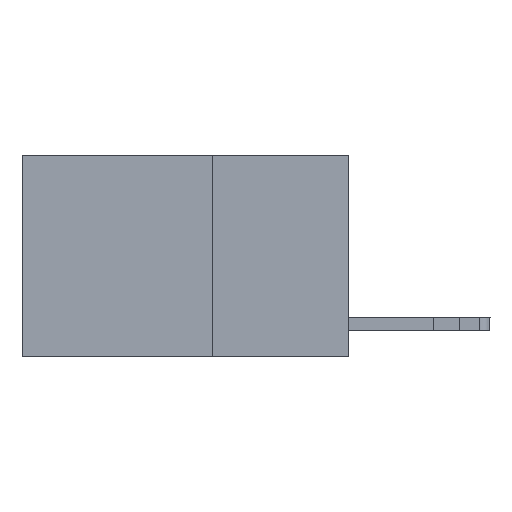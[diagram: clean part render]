
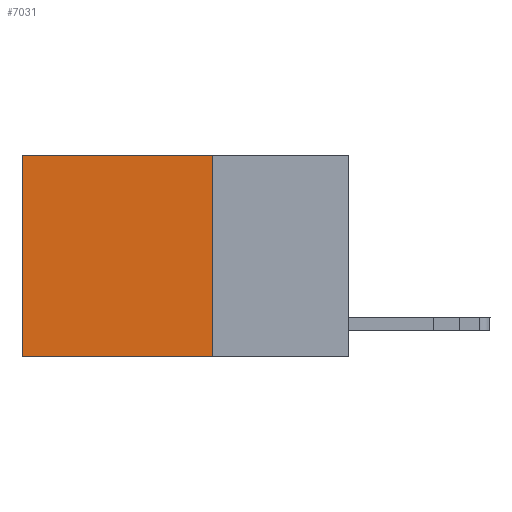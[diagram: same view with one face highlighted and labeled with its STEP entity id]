
A CAD part, left-side view. The second image highlights one B-rep face of the part: STEP entity #7031.
In plain terms, the highlighted planar face has unit normal (-1, 0, 0).
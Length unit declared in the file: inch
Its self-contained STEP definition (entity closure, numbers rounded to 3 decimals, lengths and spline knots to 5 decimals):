
#862 = DIRECTION ( 'NONE',  ( 0., 1., 0. ) ) ;
#894 = VECTOR ( 'NONE', #5470, 39.37008 ) ;
#1124 = LINE ( 'NONE', #4192, #15890 ) ;
#1819 = ORIENTED_EDGE ( 'NONE', *, *, #9313, .T. ) ;
#2173 = VERTEX_POINT ( 'NONE', #9070 ) ;
#2530 = CARTESIAN_POINT ( 'NONE',  ( 0.2625, 0.6, 0. ) ) ;
#3098 = CARTESIAN_POINT ( 'NONE',  ( 0.2625, 0.25, 0. ) ) ;
#3713 = CARTESIAN_POINT ( 'NONE',  ( 0.2625, 0.6, 0. ) ) ;
#3821 = EDGE_CURVE ( 'NONE', #17610, #4290, #5163, .T. ) ;
#4192 = CARTESIAN_POINT ( 'NONE',  ( 0.2625, 0.25, 0. ) ) ;
#4290 = VERTEX_POINT ( 'NONE', #9651 ) ;
#4427 = LINE ( 'NONE', #2530, #894 ) ;
#4977 = LINE ( 'NONE', #17897, #15807 ) ;
#5163 = LINE ( 'NONE', #5832, #18095 ) ;
#5470 = DIRECTION ( 'NONE',  ( 0., 0., -1. ) ) ;
#5767 = EDGE_CURVE ( 'NONE', #2173, #17610, #1124, .T. ) ;
#5832 = CARTESIAN_POINT ( 'NONE',  ( 0.2625, 0.25, -0.37 ) ) ;
#6005 = DIRECTION ( 'NONE',  ( 0., 0., -1. ) ) ;
#6400 = EDGE_LOOP ( 'NONE', ( #14138, #8696, #16704, #1819 ) ) ;
#7031 = ADVANCED_FACE ( 'NONE', ( #11321 ), #13071, .F. ) ;
#7268 = DIRECTION ( 'NONE',  ( 0., 1., 0. ) ) ;
#8696 = ORIENTED_EDGE ( 'NONE', *, *, #3821, .F. ) ;
#9070 = CARTESIAN_POINT ( 'NONE',  ( 0.2625, 0.25, 0. ) ) ;
#9313 = EDGE_CURVE ( 'NONE', #2173, #13031, #4977, .T. ) ;
#9651 = CARTESIAN_POINT ( 'NONE',  ( 0.2625, 0.6, -0.37 ) ) ;
#11321 = FACE_OUTER_BOUND ( 'NONE', #6400, .T. ) ;
#11364 = DIRECTION ( 'NONE',  ( 0., 0., -1. ) ) ;
#13031 = VERTEX_POINT ( 'NONE', #3713 ) ;
#13071 = PLANE ( 'NONE',  #13250 ) ;
#13250 = AXIS2_PLACEMENT_3D ( 'NONE', #3098, #14466, #6005 ) ;
#14138 = ORIENTED_EDGE ( 'NONE', *, *, #18113, .T. ) ;
#14466 = DIRECTION ( 'NONE',  ( 1., 0., 0. ) ) ;
#15807 = VECTOR ( 'NONE', #862, 39.37008 ) ;
#15890 = VECTOR ( 'NONE', #11364, 39.37008 ) ;
#16704 = ORIENTED_EDGE ( 'NONE', *, *, #5767, .F. ) ;
#17610 = VERTEX_POINT ( 'NONE', #18321 ) ;
#17897 = CARTESIAN_POINT ( 'NONE',  ( 0.2625, 0.25, 0. ) ) ;
#18095 = VECTOR ( 'NONE', #7268, 39.37008 ) ;
#18113 = EDGE_CURVE ( 'NONE', #13031, #4290, #4427, .T. ) ;
#18321 = CARTESIAN_POINT ( 'NONE',  ( 0.2625, 0.25, -0.37 ) ) ;
